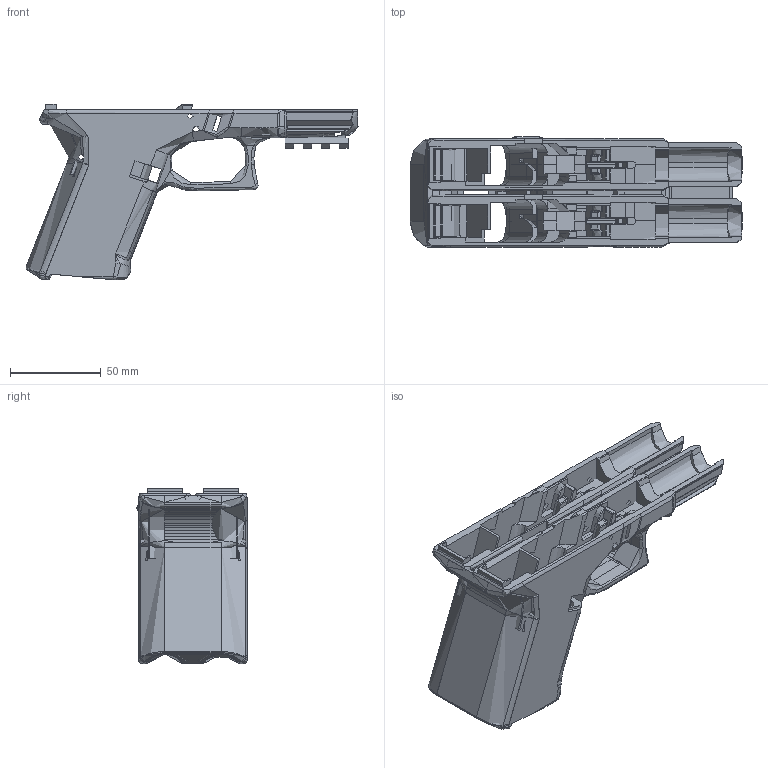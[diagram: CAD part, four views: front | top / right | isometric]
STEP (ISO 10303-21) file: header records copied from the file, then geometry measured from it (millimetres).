
FILE_DESCRIPTION(/* description */ (''),/* implementation_level */ '2;1');
FILE_NAME(/* name */ 'Glocknofsky 19 Beta v2 v8.step',/* time_stamp */ '2022-06-08T01:05:49-04:00',/* author */ (''),/* organization */ (''),/* preprocessor_version */ 'ST-DEVELOPER v19',/* originating_system */ 'Autodesk Translation Framework v11.7.0.108',/* authorisation */ '');
FILE_SCHEMA (('AUTOMOTIVE_DESIGN { 1 0 10303 214 3 1 1 }'));
Products named in the file (4): Glocknofsky 19 Beta v2; Component1; 5 Slot Picatinny Rail; Component2
Assembly tree (3 placements, depth 2):
  Glocknofsky 19 Beta v2
    Component1
    5 Slot Picatinny Rail
    Component2
Bounding box: 183.21 x 60.84 x 97.01 mm (x, y, z)
Volume: 219311.9 mm3
Topology: 19 solids, 26 shells, 2512 faces, 7056 edges, 4556 vertices
Faces by surface type: plane 1297, bspline 775, cylinder 330, torus 62, cone 24, sphere 24
Full cylindrical faces by diameter (mm): 2 x2, 3 x8, 3.2 x4, 4 x4, 24 x1
Entity records: 145011 total; most frequent: CARTESIAN_POINT 85358, ORIENTED_EDGE 14058, DIRECTION 10058, EDGE_CURVE 7029, VERTEX_POINT 4556, LINE 3858, VECTOR 3858, AXIS2_PLACEMENT_3D 3100
